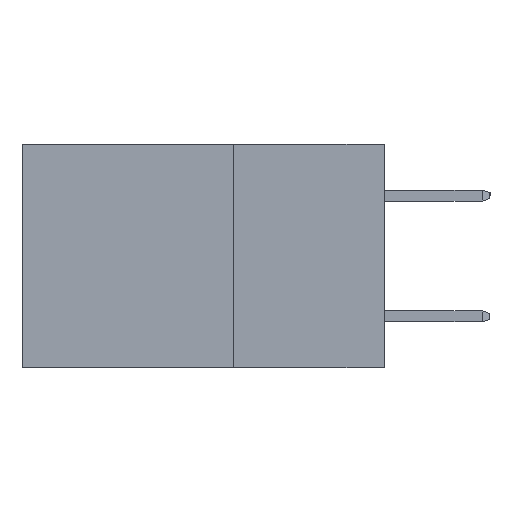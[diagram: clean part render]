
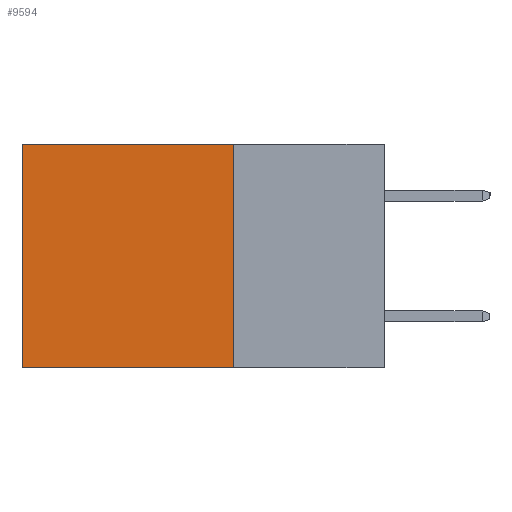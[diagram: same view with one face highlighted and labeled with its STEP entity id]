
A CAD part, left-side view. The second image highlights one B-rep face of the part: STEP entity #9594.
In plain terms, the highlighted planar face has unit normal (-1, 0, 0).
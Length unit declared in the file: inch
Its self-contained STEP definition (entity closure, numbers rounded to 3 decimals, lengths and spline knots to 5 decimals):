
#465 = CARTESIAN_POINT ( 'NONE',  ( 0.2615, 0.6, -0.37 ) ) ;
#649 = FACE_OUTER_BOUND ( 'NONE', #15209, .T. ) ;
#1527 = CARTESIAN_POINT ( 'NONE',  ( 0.2615, 0.25, 0. ) ) ;
#1556 = VERTEX_POINT ( 'NONE', #6115 ) ;
#1992 = VECTOR ( 'NONE', #6900, 39.37008 ) ;
#2285 = EDGE_CURVE ( 'NONE', #13449, #4473, #2960, .T. ) ;
#2647 = CARTESIAN_POINT ( 'NONE',  ( 0.2615, 0.6, -0.37 ) ) ;
#2960 = LINE ( 'NONE', #465, #9170 ) ;
#3194 = CARTESIAN_POINT ( 'NONE',  ( 0.2615, 0.25, -0.37 ) ) ;
#4473 = VERTEX_POINT ( 'NONE', #2647 ) ;
#4941 = EDGE_CURVE ( 'NONE', #13407, #1556, #11828, .T. ) ;
#5052 = VECTOR ( 'NONE', #12561, 39.37008 ) ;
#5244 = ORIENTED_EDGE ( 'NONE', *, *, #2285, .T. ) ;
#5556 = CARTESIAN_POINT ( 'NONE',  ( 0.2615, 0.25, -0.37 ) ) ;
#6115 = CARTESIAN_POINT ( 'NONE',  ( 0.2615, 0.25, -0.37 ) ) ;
#6592 = PLANE ( 'NONE',  #10278 ) ;
#6900 = DIRECTION ( 'NONE',  ( 0., 1., 0. ) ) ;
#7754 = LINE ( 'NONE', #13993, #5052 ) ;
#8071 = ORIENTED_EDGE ( 'NONE', *, *, #15141, .F. ) ;
#8595 = CARTESIAN_POINT ( 'NONE',  ( 0.2615, 0.6, 0. ) ) ;
#8681 = VECTOR ( 'NONE', #12971, 39.37008 ) ;
#9170 = VECTOR ( 'NONE', #12577, 39.37008 ) ;
#9594 = ADVANCED_FACE ( 'NONE', ( #649 ), #6592, .F. ) ;
#9815 = ORIENTED_EDGE ( 'NONE', *, *, #4941, .F. ) ;
#10278 = AXIS2_PLACEMENT_3D ( 'NONE', #5556, #11302, #14033 ) ;
#10575 = CARTESIAN_POINT ( 'NONE',  ( 0.2615, 0.25, 0. ) ) ;
#11302 = DIRECTION ( 'NONE',  ( 1., 0., 0. ) ) ;
#11828 = LINE ( 'NONE', #3194, #8681 ) ;
#12561 = DIRECTION ( 'NONE',  ( 0., 1., 0. ) ) ;
#12577 = DIRECTION ( 'NONE',  ( 0., 0., -1. ) ) ;
#12971 = DIRECTION ( 'NONE',  ( 0., 0., -1. ) ) ;
#13407 = VERTEX_POINT ( 'NONE', #1527 ) ;
#13449 = VERTEX_POINT ( 'NONE', #8595 ) ;
#13993 = CARTESIAN_POINT ( 'NONE',  ( 0.2615, 0.25, -0.37 ) ) ;
#14033 = DIRECTION ( 'NONE',  ( 0., 0., -1. ) ) ;
#14331 = LINE ( 'NONE', #10575, #1992 ) ;
#14878 = EDGE_CURVE ( 'NONE', #13407, #13449, #14331, .T. ) ;
#15141 = EDGE_CURVE ( 'NONE', #1556, #4473, #7754, .T. ) ;
#15209 = EDGE_LOOP ( 'NONE', ( #5244, #8071, #9815, #15226 ) ) ;
#15226 = ORIENTED_EDGE ( 'NONE', *, *, #14878, .T. ) ;
